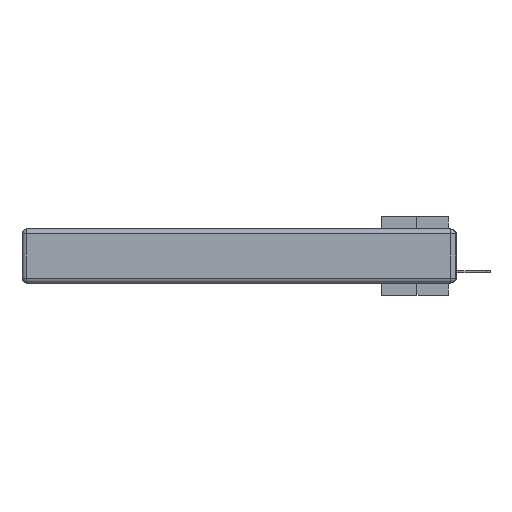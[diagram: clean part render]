
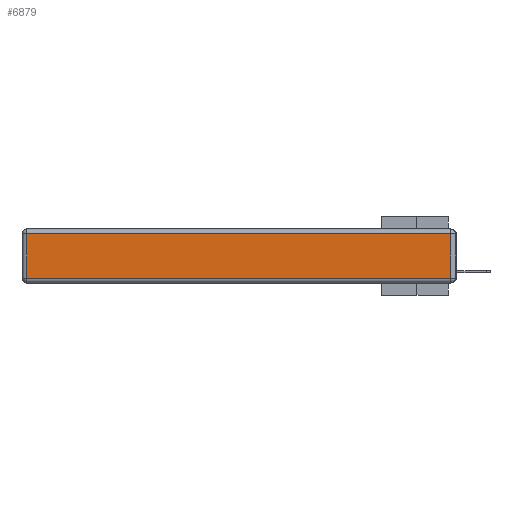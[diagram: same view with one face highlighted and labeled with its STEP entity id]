
A CAD part, left-side view. The second image highlights one B-rep face of the part: STEP entity #6879.
In plain terms, the highlighted planar face has unit normal (-1, 0, 0).
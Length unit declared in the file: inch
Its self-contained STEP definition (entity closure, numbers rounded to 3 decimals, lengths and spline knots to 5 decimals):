
#1559 = PLANE ( 'NONE',  #25860 ) ;
#1828 = VECTOR ( 'NONE', #13852, 39.37008 ) ;
#3082 = CARTESIAN_POINT ( 'NONE',  ( 0., 0.03, -0.03 ) ) ;
#3535 = CARTESIAN_POINT ( 'NONE',  ( 0., 0., -0.343 ) ) ;
#3653 = ORIENTED_EDGE ( 'NONE', *, *, #31795, .T. ) ;
#3802 = VECTOR ( 'NONE', #26971, 39.37008 ) ;
#6879 = ADVANCED_FACE ( 'NONE', ( #16491 ), #1559, .T. ) ;
#6985 = LINE ( 'NONE', #27440, #13794 ) ;
#7435 = ORIENTED_EDGE ( 'NONE', *, *, #20223, .T. ) ;
#10335 = CARTESIAN_POINT ( 'NONE',  ( 0., 2.72, -0.313 ) ) ;
#10412 = CARTESIAN_POINT ( 'NONE',  ( 0., 0.03, -0.343 ) ) ;
#10730 = VERTEX_POINT ( 'NONE', #10335 ) ;
#12759 = DIRECTION ( 'NONE',  ( 0., 0., 1. ) ) ;
#13794 = VECTOR ( 'NONE', #32603, 39.37008 ) ;
#13852 = DIRECTION ( 'NONE',  ( 0., -1., 0. ) ) ;
#15605 = CARTESIAN_POINT ( 'NONE',  ( 0., 2.72, -0.03 ) ) ;
#16491 = FACE_OUTER_BOUND ( 'NONE', #25592, .T. ) ;
#17477 = EDGE_CURVE ( 'NONE', #31055, #22267, #27907, .T. ) ;
#18303 = VERTEX_POINT ( 'NONE', #15605 ) ;
#20223 = EDGE_CURVE ( 'NONE', #18303, #10730, #32298, .T. ) ;
#21833 = DIRECTION ( 'NONE',  ( -1., 0., 0. ) ) ;
#21972 = CARTESIAN_POINT ( 'NONE',  ( 0., 2.72, -0.343 ) ) ;
#22267 = VERTEX_POINT ( 'NONE', #3082 ) ;
#23511 = LINE ( 'NONE', #25835, #1828 ) ;
#24465 = CARTESIAN_POINT ( 'NONE',  ( 0., 0.03, -0.313 ) ) ;
#25592 = EDGE_LOOP ( 'NONE', ( #3653, #30867, #28215, #7435 ) ) ;
#25835 = CARTESIAN_POINT ( 'NONE',  ( 0., 0., -0.313 ) ) ;
#25860 = AXIS2_PLACEMENT_3D ( 'NONE', #3535, #21833, #28983 ) ;
#26586 = EDGE_CURVE ( 'NONE', #22267, #18303, #6985, .T. ) ;
#26971 = DIRECTION ( 'NONE',  ( 0., 0., -1. ) ) ;
#27089 = VECTOR ( 'NONE', #12759, 39.37008 ) ;
#27440 = CARTESIAN_POINT ( 'NONE',  ( 0., 2.75, -0.03 ) ) ;
#27907 = LINE ( 'NONE', #10412, #27089 ) ;
#28215 = ORIENTED_EDGE ( 'NONE', *, *, #26586, .T. ) ;
#28983 = DIRECTION ( 'NONE',  ( 0., 0., 1. ) ) ;
#30867 = ORIENTED_EDGE ( 'NONE', *, *, #17477, .T. ) ;
#31055 = VERTEX_POINT ( 'NONE', #24465 ) ;
#31795 = EDGE_CURVE ( 'NONE', #10730, #31055, #23511, .T. ) ;
#32298 = LINE ( 'NONE', #21972, #3802 ) ;
#32603 = DIRECTION ( 'NONE',  ( 0., 1., 0. ) ) ;
